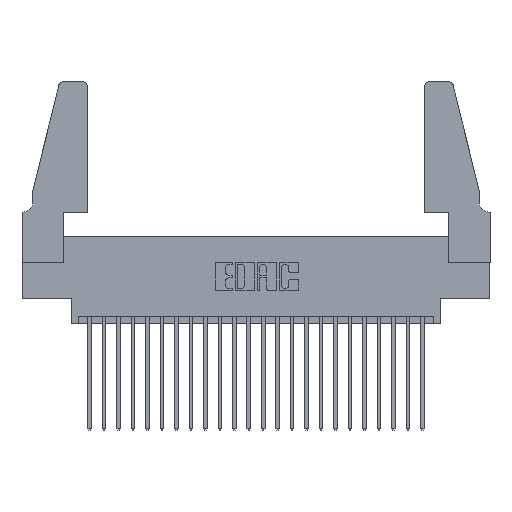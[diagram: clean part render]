
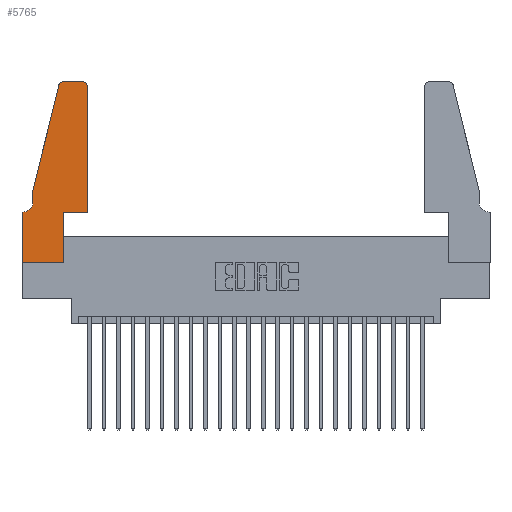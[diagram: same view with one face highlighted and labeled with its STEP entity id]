
A CAD part, top view. The second image highlights one B-rep face of the part: STEP entity #5765.
In plain terms, the highlighted planar face has unit normal (0, 0, 1).
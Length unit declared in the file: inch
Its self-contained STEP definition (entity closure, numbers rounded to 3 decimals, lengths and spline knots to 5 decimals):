
#80 = EDGE_CURVE ( 'NONE', #22709, #15732, #22809, .T. ) ;
#174 = CARTESIAN_POINT ( 'NONE',  ( 0.25487, 1.22718, 0.37 ) ) ;
#464 = DIRECTION ( 'NONE',  ( -1., 0., 0. ) ) ;
#1306 = EDGE_CURVE ( 'NONE', #3642, #12317, #12931, .T. ) ;
#1499 = CARTESIAN_POINT ( 'NONE',  ( 0.4505, 1.22, 0.37 ) ) ;
#1943 = LINE ( 'NONE', #3575, #6851 ) ;
#1980 = ORIENTED_EDGE ( 'NONE', *, *, #13388, .T. ) ;
#2444 = VERTEX_POINT ( 'NONE', #174 ) ;
#2561 = LINE ( 'NONE', #16167, #16486 ) ;
#2647 = VECTOR ( 'NONE', #12200, 39.37008 ) ;
#2703 = VECTOR ( 'NONE', #14212, 39.37008 ) ;
#2961 = ORIENTED_EDGE ( 'NONE', *, *, #12481, .T. ) ;
#3111 = VERTEX_POINT ( 'NONE', #4120 ) ;
#3434 = ORIENTED_EDGE ( 'NONE', *, *, #5008, .T. ) ;
#3533 = VERTEX_POINT ( 'NONE', #1499 ) ;
#3575 = CARTESIAN_POINT ( 'NONE',  ( 0.2865, 0.35, 0.37 ) ) ;
#3642 = VERTEX_POINT ( 'NONE', #23533 ) ;
#4087 = CARTESIAN_POINT ( 'NONE',  ( 0.4505, 0.35, 0.37 ) ) ;
#4120 = CARTESIAN_POINT ( 'NONE',  ( 0.284, 1.25, 0.37 ) ) ;
#4581 = CARTESIAN_POINT ( 'NONE',  ( 0.4505, 0.35, 0.37 ) ) ;
#5008 = EDGE_CURVE ( 'NONE', #6267, #22709, #1943, .T. ) ;
#5379 = AXIS2_PLACEMENT_3D ( 'NONE', #20356, #22161, #11370 ) ;
#5384 = FACE_OUTER_BOUND ( 'NONE', #13264, .T. ) ;
#5560 = CARTESIAN_POINT ( 'NONE',  ( 0.2865, 0., 0.37 ) ) ;
#5593 = ORIENTED_EDGE ( 'NONE', *, *, #7845, .T. ) ;
#5765 = ADVANCED_FACE ( 'NONE', ( #5384 ), #7761, .T. ) ;
#6267 = VERTEX_POINT ( 'NONE', #5560 ) ;
#6518 = DIRECTION ( 'NONE',  ( 0., -1., 0. ) ) ;
#6818 = LINE ( 'NONE', #11589, #11095 ) ;
#6851 = VECTOR ( 'NONE', #12653, 39.37008 ) ;
#7239 = VERTEX_POINT ( 'NONE', #8419 ) ;
#7761 = PLANE ( 'NONE',  #5379 ) ;
#7845 = EDGE_CURVE ( 'NONE', #15732, #3533, #19166, .T. ) ;
#7850 = EDGE_CURVE ( 'NONE', #16507, #22295, #9838, .T. ) ;
#8419 = CARTESIAN_POINT ( 'NONE',  ( 0.4205, 1.25, 0.37 ) ) ;
#8486 = CIRCLE ( 'NONE', #17719, 0.03 ) ;
#8512 = DIRECTION ( 'NONE',  ( -1., 0., 0. ) ) ;
#8792 = ORIENTED_EDGE ( 'NONE', *, *, #13981, .T. ) ;
#8799 = CARTESIAN_POINT ( 'NONE',  ( 0.284, 1.22, 0.37 ) ) ;
#9045 = VECTOR ( 'NONE', #6518, 39.37008 ) ;
#9447 = DIRECTION ( 'NONE',  ( 1., 0., 0. ) ) ;
#9838 = LINE ( 'NONE', #11925, #9045 ) ;
#10036 = CARTESIAN_POINT ( 'NONE',  ( 0.4205, 1.22, 0.37 ) ) ;
#10370 = CARTESIAN_POINT ( 'NONE',  ( 0.0755, 0.5, 0.37 ) ) ;
#10604 = EDGE_CURVE ( 'NONE', #19490, #6267, #2561, .T. ) ;
#10605 = DIRECTION ( 'NONE',  ( 1., 0., 0. ) ) ;
#10759 = CARTESIAN_POINT ( 'NONE',  ( 0.0755, 0.35, 0.37 ) ) ;
#11041 = CARTESIAN_POINT ( 'NONE',  ( 0.2865, 0.35, 0.37 ) ) ;
#11095 = VECTOR ( 'NONE', #13391, 39.37008 ) ;
#11266 = CIRCLE ( 'NONE', #21151, 0.07 ) ;
#11277 = ORIENTED_EDGE ( 'NONE', *, *, #20370, .T. ) ;
#11370 = DIRECTION ( 'NONE',  ( 1., 0., 0. ) ) ;
#11510 = DIRECTION ( 'NONE',  ( 0., 0., -1. ) ) ;
#11589 = CARTESIAN_POINT ( 'NONE',  ( 0., 0., 0.37 ) ) ;
#11856 = DIRECTION ( 'NONE',  ( 1., 0., 0. ) ) ;
#11925 = CARTESIAN_POINT ( 'NONE',  ( 0.0755, 0.5, 0.37 ) ) ;
#12153 = CARTESIAN_POINT ( 'NONE',  ( 0., 0., 0.37 ) ) ;
#12200 = DIRECTION ( 'NONE',  ( -0.239, -0.971, 0. ) ) ;
#12317 = VERTEX_POINT ( 'NONE', #21910 ) ;
#12429 = LINE ( 'NONE', #21371, #2703 ) ;
#12481 = EDGE_CURVE ( 'NONE', #12317, #19490, #6818, .T. ) ;
#12653 = DIRECTION ( 'NONE',  ( 0., 1., 0. ) ) ;
#12931 = LINE ( 'NONE', #10759, #21933 ) ;
#13001 = ORIENTED_EDGE ( 'NONE', *, *, #13731, .T. ) ;
#13264 = EDGE_LOOP ( 'NONE', ( #8792, #1980, #16582, #21011, #11277, #15007, #2961, #20454, #3434, #22025, #5593, #13001 ) ) ;
#13388 = EDGE_CURVE ( 'NONE', #3111, #2444, #19475, .T. ) ;
#13391 = DIRECTION ( 'NONE',  ( 0., -1., 0. ) ) ;
#13480 = LINE ( 'NONE', #10370, #2647 ) ;
#13731 = EDGE_CURVE ( 'NONE', #3533, #7239, #8486, .T. ) ;
#13981 = EDGE_CURVE ( 'NONE', #7239, #3111, #12429, .T. ) ;
#14212 = DIRECTION ( 'NONE',  ( -1., 0., 0. ) ) ;
#14508 = EDGE_CURVE ( 'NONE', #2444, #16507, #13480, .T. ) ;
#15007 = ORIENTED_EDGE ( 'NONE', *, *, #1306, .T. ) ;
#15535 = DIRECTION ( 'NONE',  ( 0., 1., 0. ) ) ;
#15732 = VERTEX_POINT ( 'NONE', #4581 ) ;
#15737 = AXIS2_PLACEMENT_3D ( 'NONE', #8799, #21387, #10605 ) ;
#16167 = CARTESIAN_POINT ( 'NONE',  ( 0., 0., 0.37 ) ) ;
#16486 = VECTOR ( 'NONE', #17997, 39.37008 ) ;
#16507 = VERTEX_POINT ( 'NONE', #17850 ) ;
#16582 = ORIENTED_EDGE ( 'NONE', *, *, #14508, .T. ) ;
#17719 = AXIS2_PLACEMENT_3D ( 'NONE', #10036, #22613, #11856 ) ;
#17850 = CARTESIAN_POINT ( 'NONE',  ( 0.0755, 0.5, 0.37 ) ) ;
#17997 = DIRECTION ( 'NONE',  ( 1., 0., 0. ) ) ;
#18604 = VECTOR ( 'NONE', #15535, 39.37008 ) ;
#19166 = LINE ( 'NONE', #22693, #18604 ) ;
#19475 = CIRCLE ( 'NONE', #15737, 0.03 ) ;
#19490 = VERTEX_POINT ( 'NONE', #12153 ) ;
#20356 = CARTESIAN_POINT ( 'NONE',  ( 0., 0.35, 0.37 ) ) ;
#20370 = EDGE_CURVE ( 'NONE', #22295, #3642, #11266, .T. ) ;
#20454 = ORIENTED_EDGE ( 'NONE', *, *, #10604, .T. ) ;
#21011 = ORIENTED_EDGE ( 'NONE', *, *, #7850, .T. ) ;
#21151 = AXIS2_PLACEMENT_3D ( 'NONE', #22279, #11510, #464 ) ;
#21371 = CARTESIAN_POINT ( 'NONE',  ( 0.2605, 1.25, 0.37 ) ) ;
#21387 = DIRECTION ( 'NONE',  ( 0., 0., 1. ) ) ;
#21712 = VECTOR ( 'NONE', #9447, 39.37008 ) ;
#21910 = CARTESIAN_POINT ( 'NONE',  ( 0., 0.35, 0.37 ) ) ;
#21933 = VECTOR ( 'NONE', #8512, 39.37008 ) ;
#22025 = ORIENTED_EDGE ( 'NONE', *, *, #80, .T. ) ;
#22161 = DIRECTION ( 'NONE',  ( 0., 0., 1. ) ) ;
#22279 = CARTESIAN_POINT ( 'NONE',  ( 0.0055, 0.42, 0.37 ) ) ;
#22295 = VERTEX_POINT ( 'NONE', #22511 ) ;
#22511 = CARTESIAN_POINT ( 'NONE',  ( 0.0755, 0.42, 0.37 ) ) ;
#22613 = DIRECTION ( 'NONE',  ( 0., 0., 1. ) ) ;
#22693 = CARTESIAN_POINT ( 'NONE',  ( 0.4505, 0.35, 0.37 ) ) ;
#22709 = VERTEX_POINT ( 'NONE', #11041 ) ;
#22809 = LINE ( 'NONE', #4087, #21712 ) ;
#23533 = CARTESIAN_POINT ( 'NONE',  ( 0.0055, 0.35, 0.37 ) ) ;
